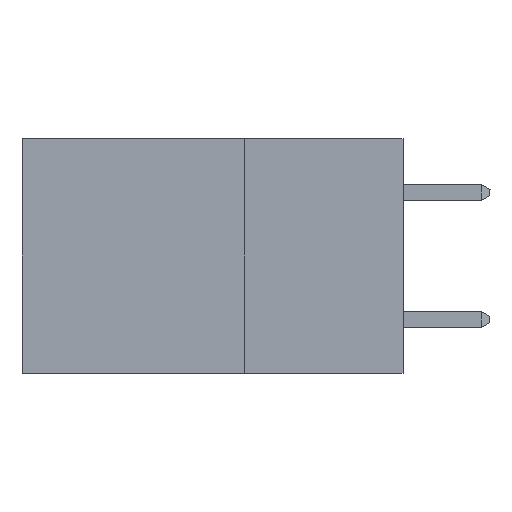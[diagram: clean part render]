
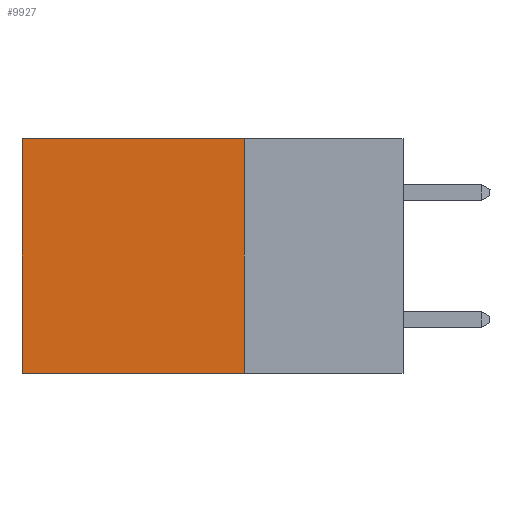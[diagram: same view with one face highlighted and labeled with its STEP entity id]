
A CAD part, left-side view. The second image highlights one B-rep face of the part: STEP entity #9927.
In plain terms, the highlighted planar face has unit normal (-1, 0, 0).
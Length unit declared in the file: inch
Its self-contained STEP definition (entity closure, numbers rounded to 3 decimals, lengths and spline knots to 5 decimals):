
#367 = EDGE_CURVE ( 'NONE', #3567, #4356, #9238, .T. ) ;
#434 = PLANE ( 'NONE',  #5312 ) ;
#1024 = CARTESIAN_POINT ( 'NONE',  ( 0.2875, 0.25, 0. ) ) ;
#1345 = VECTOR ( 'NONE', #9384, 39.37008 ) ;
#1484 = DIRECTION ( 'NONE',  ( 0., 0., -1. ) ) ;
#1546 = VECTOR ( 'NONE', #2906, 39.37008 ) ;
#2212 = CARTESIAN_POINT ( 'NONE',  ( 0.2875, 0.25, -0.37 ) ) ;
#2906 = DIRECTION ( 'NONE',  ( 0., 0., -1. ) ) ;
#3567 = VERTEX_POINT ( 'NONE', #7420 ) ;
#4355 = CARTESIAN_POINT ( 'NONE',  ( 0.2875, 0.25, 0. ) ) ;
#4356 = VERTEX_POINT ( 'NONE', #10259 ) ;
#4546 = VECTOR ( 'NONE', #7228, 39.37008 ) ;
#4629 = ORIENTED_EDGE ( 'NONE', *, *, #367, .F. ) ;
#4783 = EDGE_CURVE ( 'NONE', #10280, #11157, #7408, .T. ) ;
#4925 = ORIENTED_EDGE ( 'NONE', *, *, #5772, .F. ) ;
#5312 = AXIS2_PLACEMENT_3D ( 'NONE', #4355, #7234, #1484 ) ;
#5772 = EDGE_CURVE ( 'NONE', #10280, #3567, #9126, .T. ) ;
#5929 = FACE_OUTER_BOUND ( 'NONE', #6213, .T. ) ;
#6152 = CARTESIAN_POINT ( 'NONE',  ( 0.2875, 0.25, 0. ) ) ;
#6213 = EDGE_LOOP ( 'NONE', ( #11640, #4629, #4925, #9860 ) ) ;
#7228 = DIRECTION ( 'NONE',  ( 0., 0., -1. ) ) ;
#7234 = DIRECTION ( 'NONE',  ( 1., 0., 0. ) ) ;
#7408 = LINE ( 'NONE', #6152, #11886 ) ;
#7420 = CARTESIAN_POINT ( 'NONE',  ( 0.2875, 0.25, -0.37 ) ) ;
#7736 = DIRECTION ( 'NONE',  ( 0., 1., 0. ) ) ;
#8224 = EDGE_CURVE ( 'NONE', #11157, #4356, #9214, .T. ) ;
#9126 = LINE ( 'NONE', #9514, #1546 ) ;
#9214 = LINE ( 'NONE', #11720, #4546 ) ;
#9238 = LINE ( 'NONE', #2212, #1345 ) ;
#9384 = DIRECTION ( 'NONE',  ( 0., 1., 0. ) ) ;
#9514 = CARTESIAN_POINT ( 'NONE',  ( 0.2875, 0.25, 0. ) ) ;
#9860 = ORIENTED_EDGE ( 'NONE', *, *, #4783, .T. ) ;
#9927 = ADVANCED_FACE ( 'NONE', ( #5929 ), #434, .F. ) ;
#10259 = CARTESIAN_POINT ( 'NONE',  ( 0.2875, 0.6, -0.37 ) ) ;
#10280 = VERTEX_POINT ( 'NONE', #1024 ) ;
#11157 = VERTEX_POINT ( 'NONE', #11626 ) ;
#11626 = CARTESIAN_POINT ( 'NONE',  ( 0.2875, 0.6, 0. ) ) ;
#11640 = ORIENTED_EDGE ( 'NONE', *, *, #8224, .T. ) ;
#11720 = CARTESIAN_POINT ( 'NONE',  ( 0.2875, 0.6, 0. ) ) ;
#11886 = VECTOR ( 'NONE', #7736, 39.37008 ) ;
